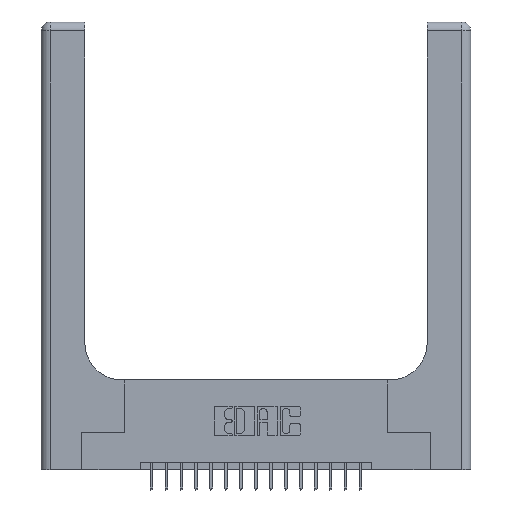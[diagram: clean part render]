
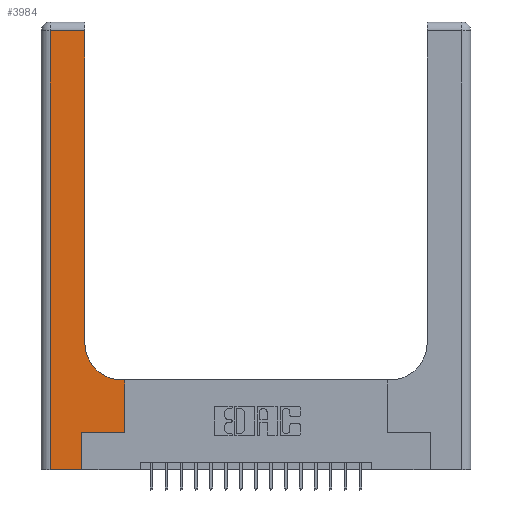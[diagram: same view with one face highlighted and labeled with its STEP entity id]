
A CAD part, top view. The second image highlights one B-rep face of the part: STEP entity #3984.
In plain terms, the highlighted planar face has unit normal (0, 0, 1).
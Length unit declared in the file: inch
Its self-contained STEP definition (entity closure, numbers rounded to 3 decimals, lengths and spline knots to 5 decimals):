
#126 = CARTESIAN_POINT ( 'NONE',  ( 0.269, 0., 0.37 ) ) ;
#304 = VERTEX_POINT ( 'NONE', #9652 ) ;
#447 = FACE_OUTER_BOUND ( 'NONE', #7671, .T. ) ;
#749 = EDGE_CURVE ( 'NONE', #7864, #20344, #3862, .T. ) ;
#1671 = ORIENTED_EDGE ( 'NONE', *, *, #4625, .T. ) ;
#2168 = EDGE_CURVE ( 'NONE', #20344, #15630, #14114, .T. ) ;
#2186 = DIRECTION ( 'NONE',  ( 0., 1., 0. ) ) ;
#2362 = VERTEX_POINT ( 'NONE', #126 ) ;
#2643 = LINE ( 'NONE', #18261, #11506 ) ;
#2777 = CIRCLE ( 'NONE', #17173, 0.25 ) ;
#2798 = DIRECTION ( 'NONE',  ( -1., 0., 0. ) ) ;
#3094 = ORIENTED_EDGE ( 'NONE', *, *, #9477, .T. ) ;
#3353 = CARTESIAN_POINT ( 'NONE',  ( 0.2915, 0.85, 0.37 ) ) ;
#3632 = ORIENTED_EDGE ( 'NONE', *, *, #749, .T. ) ;
#3678 = CARTESIAN_POINT ( 'NONE',  ( 0., 3., 0.37 ) ) ;
#3745 = CARTESIAN_POINT ( 'NONE',  ( 0.5585, 0.6, 0.37 ) ) ;
#3862 = LINE ( 'NONE', #6964, #11439 ) ;
#3910 = DIRECTION ( 'NONE',  ( -1., 0., 0. ) ) ;
#3984 = ADVANCED_FACE ( 'NONE', ( #447 ), #18029, .F. ) ;
#4095 = VECTOR ( 'NONE', #9192, 39.37008 ) ;
#4243 = LINE ( 'NONE', #7655, #5957 ) ;
#4462 = CARTESIAN_POINT ( 'NONE',  ( 0., 0., 0.37 ) ) ;
#4625 = EDGE_CURVE ( 'NONE', #16443, #7864, #2777, .T. ) ;
#5239 = CARTESIAN_POINT ( 'NONE',  ( 0.5415, 0.85, 0.37 ) ) ;
#5441 = AXIS2_PLACEMENT_3D ( 'NONE', #3678, #17053, #2798 ) ;
#5893 = DIRECTION ( 'NONE',  ( 0., 1., 0. ) ) ;
#5957 = VECTOR ( 'NONE', #18880, 39.37008 ) ;
#6020 = ORIENTED_EDGE ( 'NONE', *, *, #14593, .T. ) ;
#6210 = EDGE_CURVE ( 'NONE', #11530, #2362, #12333, .T. ) ;
#6463 = DIRECTION ( 'NONE',  ( 1., 0., 0. ) ) ;
#6964 = CARTESIAN_POINT ( 'NONE',  ( 0.2915, 3., 0.37 ) ) ;
#7188 = CARTESIAN_POINT ( 'NONE',  ( 0.2915, 2.94, 0.37 ) ) ;
#7559 = CARTESIAN_POINT ( 'NONE',  ( 0.269, 0., 0.37 ) ) ;
#7655 = CARTESIAN_POINT ( 'NONE',  ( 0.5585, 0.25, 0.37 ) ) ;
#7671 = EDGE_LOOP ( 'NONE', ( #3632, #13132, #13785, #11161, #9712, #6020, #13154, #3094, #1671 ) ) ;
#7864 = VERTEX_POINT ( 'NONE', #3353 ) ;
#8892 = VECTOR ( 'NONE', #5893, 39.37008 ) ;
#8975 = VECTOR ( 'NONE', #6463, 39.37008 ) ;
#9192 = DIRECTION ( 'NONE',  ( -1., 0., 0. ) ) ;
#9477 = EDGE_CURVE ( 'NONE', #20093, #16443, #2643, .T. ) ;
#9652 = CARTESIAN_POINT ( 'NONE',  ( 0.5585, 0.25, 0.37 ) ) ;
#9712 = ORIENTED_EDGE ( 'NONE', *, *, #10129, .T. ) ;
#9729 = DIRECTION ( 'NONE',  ( 0., 0., -1. ) ) ;
#9846 = VECTOR ( 'NONE', #17230, 39.37008 ) ;
#10129 = EDGE_CURVE ( 'NONE', #2362, #12107, #13636, .T. ) ;
#10897 = CARTESIAN_POINT ( 'NONE',  ( 0.269, 0.25, 0.37 ) ) ;
#11161 = ORIENTED_EDGE ( 'NONE', *, *, #6210, .T. ) ;
#11439 = VECTOR ( 'NONE', #2186, 39.37008 ) ;
#11506 = VECTOR ( 'NONE', #3910, 39.37008 ) ;
#11530 = VERTEX_POINT ( 'NONE', #19903 ) ;
#12107 = VERTEX_POINT ( 'NONE', #10897 ) ;
#12333 = LINE ( 'NONE', #4462, #9846 ) ;
#13132 = ORIENTED_EDGE ( 'NONE', *, *, #2168, .T. ) ;
#13154 = ORIENTED_EDGE ( 'NONE', *, *, #14197, .T. ) ;
#13636 = LINE ( 'NONE', #7559, #8892 ) ;
#13785 = ORIENTED_EDGE ( 'NONE', *, *, #17314, .T. ) ;
#14114 = LINE ( 'NONE', #17197, #4095 ) ;
#14197 = EDGE_CURVE ( 'NONE', #304, #20093, #4243, .T. ) ;
#14407 = LINE ( 'NONE', #19251, #8975 ) ;
#14593 = EDGE_CURVE ( 'NONE', #12107, #304, #14407, .T. ) ;
#15024 = CARTESIAN_POINT ( 'NONE',  ( 0.06, 2.94, 0.37 ) ) ;
#15630 = VERTEX_POINT ( 'NONE', #15024 ) ;
#16443 = VERTEX_POINT ( 'NONE', #19388 ) ;
#17048 = CARTESIAN_POINT ( 'NONE',  ( 0.06, 3., 0.37 ) ) ;
#17053 = DIRECTION ( 'NONE',  ( 0., 0., -1. ) ) ;
#17173 = AXIS2_PLACEMENT_3D ( 'NONE', #5239, #9729, #18139 ) ;
#17197 = CARTESIAN_POINT ( 'NONE',  ( 0., 2.94, 0.37 ) ) ;
#17230 = DIRECTION ( 'NONE',  ( 1., 0., 0. ) ) ;
#17314 = EDGE_CURVE ( 'NONE', #15630, #11530, #20289, .T. ) ;
#18029 = PLANE ( 'NONE',  #5441 ) ;
#18139 = DIRECTION ( 'NONE',  ( 1., 0., 0. ) ) ;
#18261 = CARTESIAN_POINT ( 'NONE',  ( 0.2915, 0.6, 0.37 ) ) ;
#18711 = VECTOR ( 'NONE', #18730, 39.37008 ) ;
#18730 = DIRECTION ( 'NONE',  ( 0., -1., 0. ) ) ;
#18880 = DIRECTION ( 'NONE',  ( 0., 1., 0. ) ) ;
#19251 = CARTESIAN_POINT ( 'NONE',  ( 0.269, 0.25, 0.37 ) ) ;
#19388 = CARTESIAN_POINT ( 'NONE',  ( 0.5415, 0.6, 0.37 ) ) ;
#19903 = CARTESIAN_POINT ( 'NONE',  ( 0.06, 0., 0.37 ) ) ;
#20093 = VERTEX_POINT ( 'NONE', #3745 ) ;
#20289 = LINE ( 'NONE', #17048, #18711 ) ;
#20344 = VERTEX_POINT ( 'NONE', #7188 ) ;
